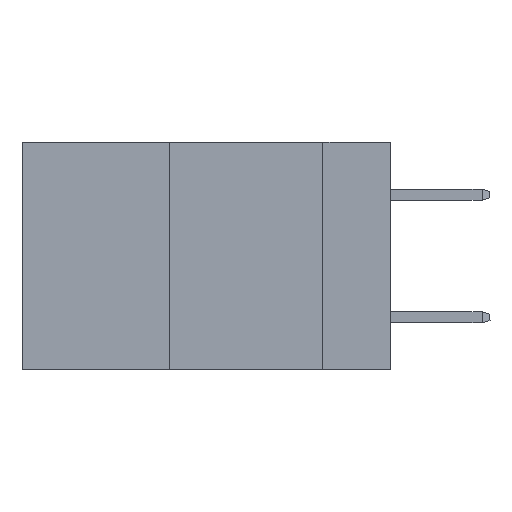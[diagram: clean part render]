
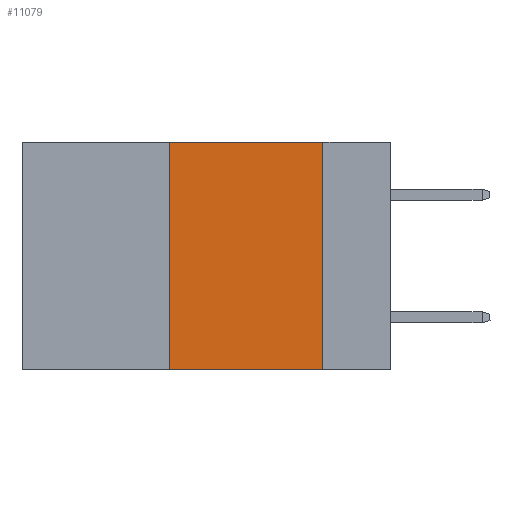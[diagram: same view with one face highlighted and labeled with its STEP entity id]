
A CAD part, left-side view. The second image highlights one B-rep face of the part: STEP entity #11079.
In plain terms, the highlighted planar face has unit normal (-1, 0, 0).
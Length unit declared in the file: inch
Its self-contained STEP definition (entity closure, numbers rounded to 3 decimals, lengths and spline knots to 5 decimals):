
#942 = EDGE_CURVE ( 'NONE', #12236, #6227, #9368, .T. ) ;
#1182 = FACE_OUTER_BOUND ( 'NONE', #7881, .T. ) ;
#1515 = ORIENTED_EDGE ( 'NONE', *, *, #3829, .F. ) ;
#2001 = ORIENTED_EDGE ( 'NONE', *, *, #3376, .F. ) ;
#2363 = LINE ( 'NONE', #13121, #6209 ) ;
#3376 = EDGE_CURVE ( 'NONE', #13636, #12236, #6089, .T. ) ;
#3383 = DIRECTION ( 'NONE',  ( 0., -1., 0. ) ) ;
#3829 = EDGE_CURVE ( 'NONE', #6227, #17233, #12958, .T. ) ;
#4605 = CARTESIAN_POINT ( 'NONE',  ( 0., 0.6, 0. ) ) ;
#5433 = ORIENTED_EDGE ( 'NONE', *, *, #942, .F. ) ;
#5738 = VECTOR ( 'NONE', #10913, 39.37008 ) ;
#6089 = LINE ( 'NONE', #12844, #16704 ) ;
#6209 = VECTOR ( 'NONE', #3383, 39.37008 ) ;
#6227 = VERTEX_POINT ( 'NONE', #14405 ) ;
#6288 = EDGE_CURVE ( 'NONE', #13636, #17233, #2363, .T. ) ;
#7130 = CARTESIAN_POINT ( 'NONE',  ( 0., 0.11, 0. ) ) ;
#7164 = DIRECTION ( 'NONE',  ( 0., 0., -1. ) ) ;
#7368 = DIRECTION ( 'NONE',  ( 1., 0., 0. ) ) ;
#7535 = AXIS2_PLACEMENT_3D ( 'NONE', #4605, #7368, #17088 ) ;
#7881 = EDGE_LOOP ( 'NONE', ( #1515, #5433, #2001, #9479 ) ) ;
#9368 = LINE ( 'NONE', #17459, #5738 ) ;
#9479 = ORIENTED_EDGE ( 'NONE', *, *, #6288, .T. ) ;
#10449 = CARTESIAN_POINT ( 'NONE',  ( 0., 0.11, -0.37 ) ) ;
#10913 = DIRECTION ( 'NONE',  ( 0., -1., 0. ) ) ;
#11079 = ADVANCED_FACE ( 'NONE', ( #1182 ), #11438, .F. ) ;
#11438 = PLANE ( 'NONE',  #7535 ) ;
#11710 = CARTESIAN_POINT ( 'NONE',  ( 0., 0.36, -0.37 ) ) ;
#12236 = VERTEX_POINT ( 'NONE', #18136 ) ;
#12786 = DIRECTION ( 'NONE',  ( 0., 0., 1. ) ) ;
#12844 = CARTESIAN_POINT ( 'NONE',  ( 0., 0.36, 0. ) ) ;
#12958 = LINE ( 'NONE', #7130, #16234 ) ;
#13121 = CARTESIAN_POINT ( 'NONE',  ( 0., 0.6, -0.37 ) ) ;
#13636 = VERTEX_POINT ( 'NONE', #11710 ) ;
#14405 = CARTESIAN_POINT ( 'NONE',  ( 0., 0.11, 0. ) ) ;
#16234 = VECTOR ( 'NONE', #7164, 39.37008 ) ;
#16704 = VECTOR ( 'NONE', #12786, 39.37008 ) ;
#17088 = DIRECTION ( 'NONE',  ( 0., 0., -1. ) ) ;
#17233 = VERTEX_POINT ( 'NONE', #10449 ) ;
#17459 = CARTESIAN_POINT ( 'NONE',  ( 0., 0.6, 0. ) ) ;
#18136 = CARTESIAN_POINT ( 'NONE',  ( 0., 0.36, 0. ) ) ;
